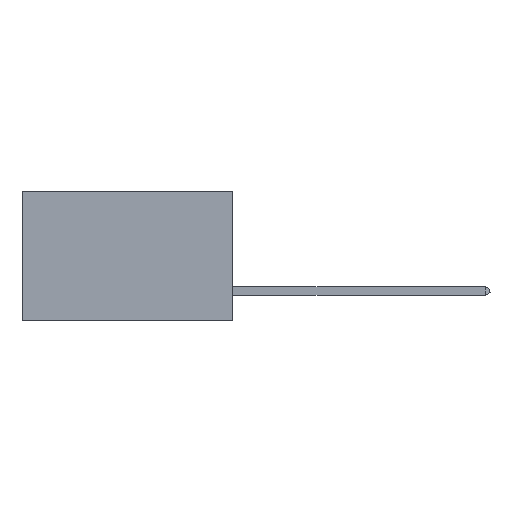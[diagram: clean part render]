
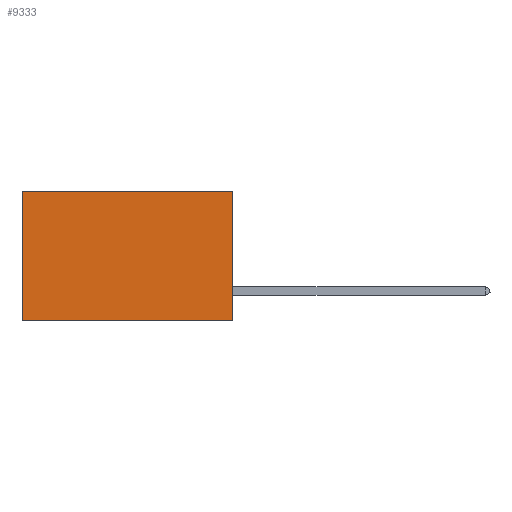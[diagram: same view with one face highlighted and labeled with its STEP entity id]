
A CAD part, left-side view. The second image highlights one B-rep face of the part: STEP entity #9333.
In plain terms, the highlighted planar face has unit normal (-1, 0, 0).
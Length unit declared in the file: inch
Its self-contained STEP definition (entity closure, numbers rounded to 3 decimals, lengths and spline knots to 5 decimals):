
#958 = LINE ( 'NONE', #16325, #13670 ) ;
#1886 = LINE ( 'NONE', #22122, #4554 ) ;
#2845 = CARTESIAN_POINT ( 'NONE',  ( 0.2875, 0., -0.37 ) ) ;
#2886 = VERTEX_POINT ( 'NONE', #27512 ) ;
#4042 = ORIENTED_EDGE ( 'NONE', *, *, #15341, .T. ) ;
#4554 = VECTOR ( 'NONE', #7483, 39.37008 ) ;
#6509 = DIRECTION ( 'NONE',  ( 0., 1., 0. ) ) ;
#6733 = ORIENTED_EDGE ( 'NONE', *, *, #25856, .T. ) ;
#6736 = ORIENTED_EDGE ( 'NONE', *, *, #7910, .F. ) ;
#7483 = DIRECTION ( 'NONE',  ( 0., 1., 0. ) ) ;
#7910 = EDGE_CURVE ( 'NONE', #25841, #21732, #958, .T. ) ;
#7944 = CARTESIAN_POINT ( 'NONE',  ( 0.2875, 0., 0. ) ) ;
#8199 = PLANE ( 'NONE',  #13229 ) ;
#8388 = DIRECTION ( 'NONE',  ( 0., 0., -1. ) ) ;
#9333 = ADVANCED_FACE ( 'NONE', ( #11915 ), #8199, .F. ) ;
#9470 = CARTESIAN_POINT ( 'NONE',  ( 0.2875, 0.6, 0. ) ) ;
#11094 = LINE ( 'NONE', #20741, #26714 ) ;
#11915 = FACE_OUTER_BOUND ( 'NONE', #23727, .T. ) ;
#12097 = VECTOR ( 'NONE', #6509, 39.37008 ) ;
#13229 = AXIS2_PLACEMENT_3D ( 'NONE', #7944, #14705, #8388 ) ;
#13670 = VECTOR ( 'NONE', #18468, 39.37008 ) ;
#14705 = DIRECTION ( 'NONE',  ( 1., 0., 0. ) ) ;
#15177 = EDGE_CURVE ( 'NONE', #21732, #2886, #23387, .T. ) ;
#15341 = EDGE_CURVE ( 'NONE', #27243, #2886, #11094, .T. ) ;
#16325 = CARTESIAN_POINT ( 'NONE',  ( 0.2875, 0., 0. ) ) ;
#18468 = DIRECTION ( 'NONE',  ( 0., 0., -1. ) ) ;
#20741 = CARTESIAN_POINT ( 'NONE',  ( 0.2875, 0.6, 0. ) ) ;
#21732 = VERTEX_POINT ( 'NONE', #27139 ) ;
#22122 = CARTESIAN_POINT ( 'NONE',  ( 0.2875, 0., 0. ) ) ;
#22727 = DIRECTION ( 'NONE',  ( 0., 0., -1. ) ) ;
#23387 = LINE ( 'NONE', #2845, #12097 ) ;
#23727 = EDGE_LOOP ( 'NONE', ( #4042, #26762, #6736, #6733 ) ) ;
#24370 = CARTESIAN_POINT ( 'NONE',  ( 0.2875, 0., 0. ) ) ;
#25841 = VERTEX_POINT ( 'NONE', #24370 ) ;
#25856 = EDGE_CURVE ( 'NONE', #25841, #27243, #1886, .T. ) ;
#26714 = VECTOR ( 'NONE', #22727, 39.37008 ) ;
#26762 = ORIENTED_EDGE ( 'NONE', *, *, #15177, .F. ) ;
#27139 = CARTESIAN_POINT ( 'NONE',  ( 0.2875, 0., -0.37 ) ) ;
#27243 = VERTEX_POINT ( 'NONE', #9470 ) ;
#27512 = CARTESIAN_POINT ( 'NONE',  ( 0.2875, 0.6, -0.37 ) ) ;
